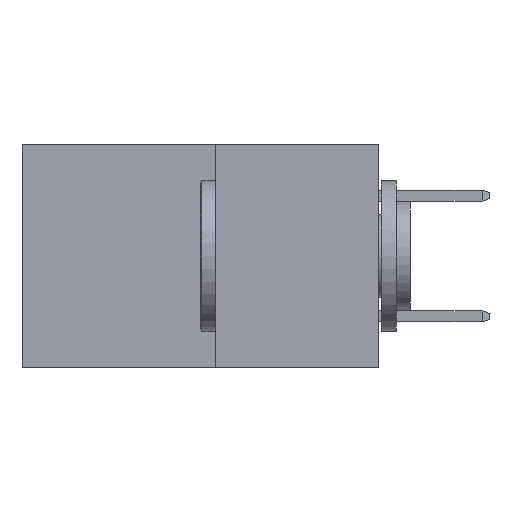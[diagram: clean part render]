
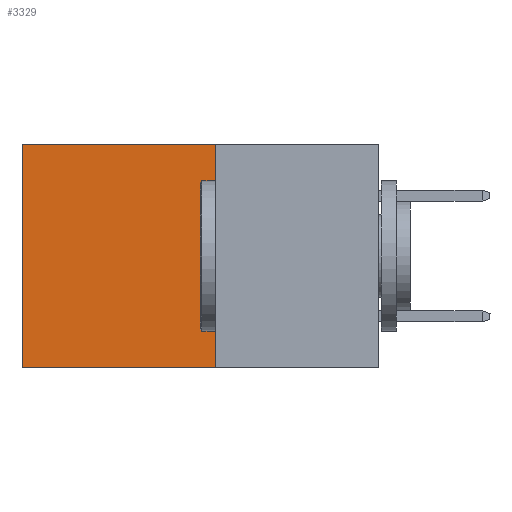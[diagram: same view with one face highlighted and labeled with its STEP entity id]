
A CAD part, left-side view. The second image highlights one B-rep face of the part: STEP entity #3329.
In plain terms, the highlighted planar face has unit normal (-1, 0, 0).
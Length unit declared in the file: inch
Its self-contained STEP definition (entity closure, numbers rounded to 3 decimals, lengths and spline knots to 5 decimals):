
#48 = LINE ( 'NONE', #5920, #9013 ) ;
#426 = ORIENTED_EDGE ( 'NONE', *, *, #5301, .F. ) ;
#539 = ORIENTED_EDGE ( 'NONE', *, *, #6584, .F. ) ;
#704 = ORIENTED_EDGE ( 'NONE', *, *, #5565, .T. ) ;
#830 = VERTEX_POINT ( 'NONE', #6073 ) ;
#1059 = VECTOR ( 'NONE', #8287, 39.37008 ) ;
#1074 = VECTOR ( 'NONE', #1404, 39.37008 ) ;
#1328 = LINE ( 'NONE', #1671, #1074 ) ;
#1404 = DIRECTION ( 'NONE',  ( 0., 0., -1. ) ) ;
#1481 = DIRECTION ( 'NONE',  ( 0., 0., -1. ) ) ;
#1671 = CARTESIAN_POINT ( 'NONE',  ( 0.277, 0.27, -0.37 ) ) ;
#2206 = VERTEX_POINT ( 'NONE', #5244 ) ;
#2353 = VECTOR ( 'NONE', #3023, 39.37008 ) ;
#2465 = AXIS2_PLACEMENT_3D ( 'NONE', #3108, #3905, #1481 ) ;
#3023 = DIRECTION ( 'NONE',  ( 0., 0., -1. ) ) ;
#3037 = CARTESIAN_POINT ( 'NONE',  ( 0.277, 0.59, -0.37 ) ) ;
#3087 = ORIENTED_EDGE ( 'NONE', *, *, #5840, .T. ) ;
#3108 = CARTESIAN_POINT ( 'NONE',  ( 0.277, 0.27, -0.37 ) ) ;
#3143 = LINE ( 'NONE', #8442, #1059 ) ;
#3329 = ADVANCED_FACE ( 'NONE', ( #3411 ), #7922, .F. ) ;
#3411 = FACE_OUTER_BOUND ( 'NONE', #3977, .T. ) ;
#3905 = DIRECTION ( 'NONE',  ( 1., 0., 0. ) ) ;
#3977 = EDGE_LOOP ( 'NONE', ( #3087, #426, #539, #704 ) ) ;
#4089 = VERTEX_POINT ( 'NONE', #7487 ) ;
#4528 = LINE ( 'NONE', #3037, #2353 ) ;
#5244 = CARTESIAN_POINT ( 'NONE',  ( 0.277, 0.27, 0. ) ) ;
#5301 = EDGE_CURVE ( 'NONE', #4089, #830, #3143, .T. ) ;
#5565 = EDGE_CURVE ( 'NONE', #2206, #6904, #48, .T. ) ;
#5840 = EDGE_CURVE ( 'NONE', #6904, #830, #4528, .T. ) ;
#5920 = CARTESIAN_POINT ( 'NONE',  ( 0.277, 0.27, 0. ) ) ;
#5962 = DIRECTION ( 'NONE',  ( 0., 1., 0. ) ) ;
#6073 = CARTESIAN_POINT ( 'NONE',  ( 0.277, 0.59, -0.37 ) ) ;
#6584 = EDGE_CURVE ( 'NONE', #2206, #4089, #1328, .T. ) ;
#6904 = VERTEX_POINT ( 'NONE', #7646 ) ;
#7487 = CARTESIAN_POINT ( 'NONE',  ( 0.277, 0.27, -0.37 ) ) ;
#7646 = CARTESIAN_POINT ( 'NONE',  ( 0.277, 0.59, 0. ) ) ;
#7922 = PLANE ( 'NONE',  #2465 ) ;
#8287 = DIRECTION ( 'NONE',  ( 0., 1., 0. ) ) ;
#8442 = CARTESIAN_POINT ( 'NONE',  ( 0.277, 0.27, -0.37 ) ) ;
#9013 = VECTOR ( 'NONE', #5962, 39.37008 ) ;
